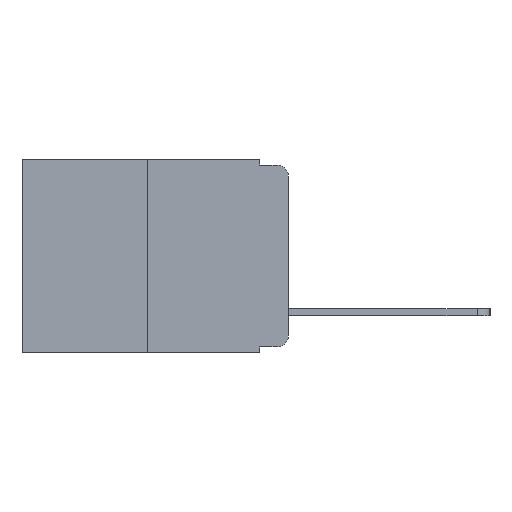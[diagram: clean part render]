
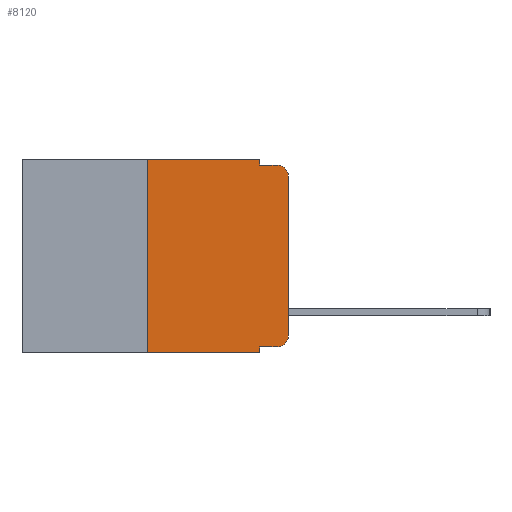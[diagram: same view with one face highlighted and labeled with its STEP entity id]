
A CAD part, left-side view. The second image highlights one B-rep face of the part: STEP entity #8120.
In plain terms, the highlighted planar face has unit normal (-1, 0, 0).
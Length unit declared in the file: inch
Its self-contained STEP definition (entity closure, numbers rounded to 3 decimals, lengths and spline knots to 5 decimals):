
#301 = VECTOR ( 'NONE', #2101, 39.37008 ) ;
#634 = VERTEX_POINT ( 'NONE', #13168 ) ;
#722 = VERTEX_POINT ( 'NONE', #21464 ) ;
#915 = LINE ( 'NONE', #20805, #18918 ) ;
#1293 = DIRECTION ( 'NONE',  ( 0., 0., 1. ) ) ;
#1915 = CARTESIAN_POINT ( 'NONE',  ( 0., 0.473, 0. ) ) ;
#2101 = DIRECTION ( 'NONE',  ( 0., -1., 0. ) ) ;
#2402 = ORIENTED_EDGE ( 'NONE', *, *, #10435, .F. ) ;
#2510 = VECTOR ( 'NONE', #11221, 39.37008 ) ;
#2585 = VERTEX_POINT ( 'NONE', #21174 ) ;
#3084 = LINE ( 'NONE', #16541, #2510 ) ;
#3120 = CARTESIAN_POINT ( 'NONE',  ( 0., 0.051, 0. ) ) ;
#3179 = EDGE_CURVE ( 'NONE', #17382, #722, #7075, .T. ) ;
#3244 = ORIENTED_EDGE ( 'NONE', *, *, #3179, .T. ) ;
#3482 = PLANE ( 'NONE',  #15248 ) ;
#3830 = ORIENTED_EDGE ( 'NONE', *, *, #15230, .T. ) ;
#4176 = VECTOR ( 'NONE', #1293, 39.37008 ) ;
#4382 = AXIS2_PLACEMENT_3D ( 'NONE', #15885, #15833, #15808 ) ;
#4429 = EDGE_CURVE ( 'NONE', #634, #17382, #5167, .T. ) ;
#4544 = CARTESIAN_POINT ( 'NONE',  ( 0., 0.02, -0.333 ) ) ;
#5059 = EDGE_CURVE ( 'NONE', #17056, #20190, #20225, .T. ) ;
#5167 = LINE ( 'NONE', #9307, #301 ) ;
#5262 = ORIENTED_EDGE ( 'NONE', *, *, #5640, .F. ) ;
#5553 = DIRECTION ( 'NONE',  ( -1., 0., 0. ) ) ;
#5587 = EDGE_LOOP ( 'NONE', ( #3830, #19811, #2402, #18997, #20686, #17307, #23145, #5262, #11711, #3244 ) ) ;
#5640 = EDGE_CURVE ( 'NONE', #634, #20190, #3084, .T. ) ;
#6085 = DIRECTION ( 'NONE',  ( 0., -1., 0. ) ) ;
#6757 = DIRECTION ( 'NONE',  ( 0., 0., -1. ) ) ;
#6824 = EDGE_CURVE ( 'NONE', #17056, #21842, #23195, .T. ) ;
#7075 = CIRCLE ( 'NONE', #4382, 0.02 ) ;
#7197 = DIRECTION ( 'NONE',  ( 0., 0., -1. ) ) ;
#7397 = AXIS2_PLACEMENT_3D ( 'NONE', #16268, #5553, #18054 ) ;
#7606 = CARTESIAN_POINT ( 'NONE',  ( 0., 0.051, -0.01 ) ) ;
#7660 = VECTOR ( 'NONE', #9411, 39.37008 ) ;
#8018 = VERTEX_POINT ( 'NONE', #8680 ) ;
#8120 = ADVANCED_FACE ( 'NONE', ( #13084 ), #3482, .F. ) ;
#8236 = LINE ( 'NONE', #7606, #7660 ) ;
#8680 = CARTESIAN_POINT ( 'NONE',  ( 0., 0.051, -0.01 ) ) ;
#8959 = DIRECTION ( 'NONE',  ( 0., -1., 0. ) ) ;
#9187 = CARTESIAN_POINT ( 'NONE',  ( 0., 0.25, 0. ) ) ;
#9227 = EDGE_CURVE ( 'NONE', #2585, #8018, #12505, .T. ) ;
#9307 = CARTESIAN_POINT ( 'NONE',  ( 0., 0.051, -0.333 ) ) ;
#9411 = DIRECTION ( 'NONE',  ( 0., -1., 0. ) ) ;
#9717 = EDGE_CURVE ( 'NONE', #21842, #2585, #20884, .T. ) ;
#10435 = EDGE_CURVE ( 'NONE', #8018, #15606, #8236, .T. ) ;
#11221 = DIRECTION ( 'NONE',  ( 0., 0., -1. ) ) ;
#11711 = ORIENTED_EDGE ( 'NONE', *, *, #4429, .T. ) ;
#11931 = VECTOR ( 'NONE', #8959, 39.37008 ) ;
#12505 = LINE ( 'NONE', #3120, #21449 ) ;
#12525 = CARTESIAN_POINT ( 'NONE',  ( 0., 0.473, 0. ) ) ;
#13084 = FACE_OUTER_BOUND ( 'NONE', #5587, .T. ) ;
#13168 = CARTESIAN_POINT ( 'NONE',  ( 0., 0.051, -0.333 ) ) ;
#13693 = DIRECTION ( 'NONE',  ( 0., 0., 1. ) ) ;
#13944 = VERTEX_POINT ( 'NONE', #21333 ) ;
#14016 = EDGE_CURVE ( 'NONE', #13944, #15606, #16990, .T. ) ;
#15230 = EDGE_CURVE ( 'NONE', #722, #13944, #915, .T. ) ;
#15248 = AXIS2_PLACEMENT_3D ( 'NONE', #12525, #17922, #7197 ) ;
#15417 = CARTESIAN_POINT ( 'NONE',  ( 0., 0.051, -0.343 ) ) ;
#15491 = VECTOR ( 'NONE', #6085, 39.37008 ) ;
#15606 = VERTEX_POINT ( 'NONE', #18287 ) ;
#15808 = DIRECTION ( 'NONE',  ( 0., 0., -1. ) ) ;
#15833 = DIRECTION ( 'NONE',  ( -1., 0., 0. ) ) ;
#15885 = CARTESIAN_POINT ( 'NONE',  ( 0., 0.02, -0.313 ) ) ;
#16268 = CARTESIAN_POINT ( 'NONE',  ( 0., 0.02, -0.03 ) ) ;
#16541 = CARTESIAN_POINT ( 'NONE',  ( 0., 0.051, 0. ) ) ;
#16808 = CARTESIAN_POINT ( 'NONE',  ( 0., 0.473, -0.343 ) ) ;
#16990 = CIRCLE ( 'NONE', #7397, 0.02 ) ;
#17056 = VERTEX_POINT ( 'NONE', #19645 ) ;
#17307 = ORIENTED_EDGE ( 'NONE', *, *, #6824, .F. ) ;
#17382 = VERTEX_POINT ( 'NONE', #4544 ) ;
#17922 = DIRECTION ( 'NONE',  ( 1., 0., 0. ) ) ;
#18054 = DIRECTION ( 'NONE',  ( 0., 0., -1. ) ) ;
#18287 = CARTESIAN_POINT ( 'NONE',  ( 0., 0.02, -0.01 ) ) ;
#18918 = VECTOR ( 'NONE', #13693, 39.37008 ) ;
#18997 = ORIENTED_EDGE ( 'NONE', *, *, #9227, .F. ) ;
#19645 = CARTESIAN_POINT ( 'NONE',  ( 0., 0.25, -0.343 ) ) ;
#19811 = ORIENTED_EDGE ( 'NONE', *, *, #14016, .T. ) ;
#20190 = VERTEX_POINT ( 'NONE', #15417 ) ;
#20225 = LINE ( 'NONE', #16808, #15491 ) ;
#20686 = ORIENTED_EDGE ( 'NONE', *, *, #9717, .F. ) ;
#20805 = CARTESIAN_POINT ( 'NONE',  ( 0., 0., 0. ) ) ;
#20884 = LINE ( 'NONE', #1915, #11931 ) ;
#21024 = CARTESIAN_POINT ( 'NONE',  ( 0., 0.25, 0. ) ) ;
#21174 = CARTESIAN_POINT ( 'NONE',  ( 0., 0.051, 0. ) ) ;
#21333 = CARTESIAN_POINT ( 'NONE',  ( 0., 0., -0.03 ) ) ;
#21449 = VECTOR ( 'NONE', #6757, 39.37008 ) ;
#21464 = CARTESIAN_POINT ( 'NONE',  ( 0., 0., -0.313 ) ) ;
#21842 = VERTEX_POINT ( 'NONE', #9187 ) ;
#23145 = ORIENTED_EDGE ( 'NONE', *, *, #5059, .T. ) ;
#23195 = LINE ( 'NONE', #21024, #4176 ) ;
